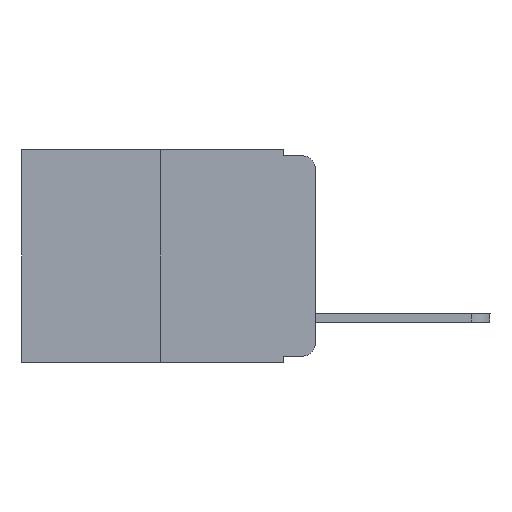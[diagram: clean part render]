
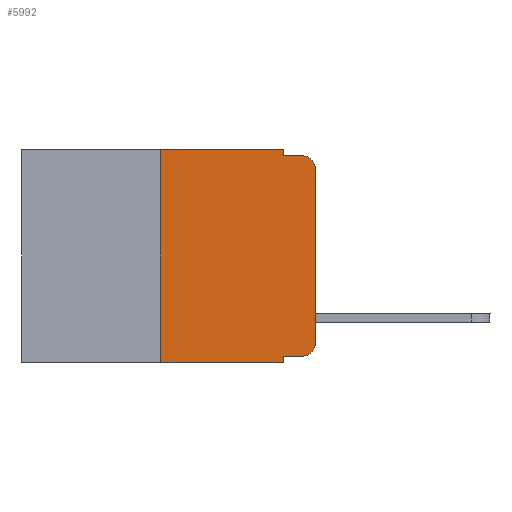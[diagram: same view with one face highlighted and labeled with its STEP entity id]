
A CAD part, left-side view. The second image highlights one B-rep face of the part: STEP entity #5992.
In plain terms, the highlighted planar face has unit normal (-1, 0, 0).
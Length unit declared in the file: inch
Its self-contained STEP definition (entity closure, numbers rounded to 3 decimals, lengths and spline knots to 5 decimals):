
#54 = VECTOR ( 'NONE', #4300, 39.37008 ) ;
#145 = VECTOR ( 'NONE', #15289, 39.37008 ) ;
#254 = PLANE ( 'NONE',  #7755 ) ;
#296 = LINE ( 'NONE', #3203, #15888 ) ;
#339 = VECTOR ( 'NONE', #8221, 39.37008 ) ;
#376 = LINE ( 'NONE', #16861, #54 ) ;
#818 = CARTESIAN_POINT ( 'NONE',  ( 0., 0.051, 0. ) ) ;
#843 = CARTESIAN_POINT ( 'NONE',  ( 0., 0.25, 0. ) ) ;
#1325 = CARTESIAN_POINT ( 'NONE',  ( 0., 0.473, 0. ) ) ;
#1671 = VERTEX_POINT ( 'NONE', #8772 ) ;
#1815 = CARTESIAN_POINT ( 'NONE',  ( 0., 0., 0. ) ) ;
#2217 = VERTEX_POINT ( 'NONE', #7642 ) ;
#2383 = ORIENTED_EDGE ( 'NONE', *, *, #7531, .F. ) ;
#2598 = CARTESIAN_POINT ( 'NONE',  ( 0., 0.02, -0.03 ) ) ;
#2731 = EDGE_CURVE ( 'NONE', #16089, #1671, #296, .T. ) ;
#2764 = CARTESIAN_POINT ( 'NONE',  ( 0., 0.051, -0.333 ) ) ;
#2862 = ORIENTED_EDGE ( 'NONE', *, *, #13841, .F. ) ;
#2972 = ORIENTED_EDGE ( 'NONE', *, *, #16739, .T. ) ;
#2994 = CARTESIAN_POINT ( 'NONE',  ( 0., 0.051, -0.01 ) ) ;
#3203 = CARTESIAN_POINT ( 'NONE',  ( 0., 0.051, -0.333 ) ) ;
#3893 = EDGE_CURVE ( 'NONE', #2217, #14074, #13773, .T. ) ;
#4105 = VERTEX_POINT ( 'NONE', #6702 ) ;
#4200 = CARTESIAN_POINT ( 'NONE',  ( 0., 0., -0.03 ) ) ;
#4300 = DIRECTION ( 'NONE',  ( 0., 0., -1. ) ) ;
#4451 = CARTESIAN_POINT ( 'NONE',  ( 0., 0.473, 0. ) ) ;
#4842 = LINE ( 'NONE', #1815, #11872 ) ;
#4880 = VERTEX_POINT ( 'NONE', #8976 ) ;
#5823 = EDGE_CURVE ( 'NONE', #4105, #11943, #7794, .T. ) ;
#5889 = DIRECTION ( 'NONE',  ( 0., -1., 0. ) ) ;
#5992 = ADVANCED_FACE ( 'NONE', ( #12905 ), #254, .F. ) ;
#6702 = CARTESIAN_POINT ( 'NONE',  ( 0., 0.051, 0. ) ) ;
#6737 = ORIENTED_EDGE ( 'NONE', *, *, #5823, .F. ) ;
#6950 = EDGE_LOOP ( 'NONE', ( #2972, #15024, #8803, #6737, #2862, #14785, #15676, #2383, #9348, #11802 ) ) ;
#6998 = DIRECTION ( 'NONE',  ( 0., 0., -1. ) ) ;
#7228 = DIRECTION ( 'NONE',  ( 0., 0., -1. ) ) ;
#7283 = DIRECTION ( 'NONE',  ( 0., -1., 0. ) ) ;
#7531 = EDGE_CURVE ( 'NONE', #16089, #12881, #376, .T. ) ;
#7642 = CARTESIAN_POINT ( 'NONE',  ( 0., 0.25, -0.343 ) ) ;
#7755 = AXIS2_PLACEMENT_3D ( 'NONE', #4451, #10089, #14267 ) ;
#7794 = LINE ( 'NONE', #818, #145 ) ;
#8005 = EDGE_CURVE ( 'NONE', #11943, #13350, #15561, .T. ) ;
#8221 = DIRECTION ( 'NONE',  ( 0., -1., 0. ) ) ;
#8237 = AXIS2_PLACEMENT_3D ( 'NONE', #8995, #8810, #7228 ) ;
#8254 = AXIS2_PLACEMENT_3D ( 'NONE', #2598, #13702, #6998 ) ;
#8705 = DIRECTION ( 'NONE',  ( 0., -1., 0. ) ) ;
#8756 = VECTOR ( 'NONE', #12595, 39.37008 ) ;
#8772 = CARTESIAN_POINT ( 'NONE',  ( 0., 0.02, -0.333 ) ) ;
#8803 = ORIENTED_EDGE ( 'NONE', *, *, #8005, .F. ) ;
#8810 = DIRECTION ( 'NONE',  ( -1., 0., 0. ) ) ;
#8976 = CARTESIAN_POINT ( 'NONE',  ( 0., 0., -0.313 ) ) ;
#8995 = CARTESIAN_POINT ( 'NONE',  ( 0., 0.02, -0.313 ) ) ;
#9348 = ORIENTED_EDGE ( 'NONE', *, *, #2731, .T. ) ;
#9381 = CARTESIAN_POINT ( 'NONE',  ( 0., 0.051, -0.343 ) ) ;
#9615 = EDGE_CURVE ( 'NONE', #2217, #12881, #16649, .T. ) ;
#9812 = CARTESIAN_POINT ( 'NONE',  ( 0., 0.02, -0.01 ) ) ;
#10089 = DIRECTION ( 'NONE',  ( 1., 0., 0. ) ) ;
#10105 = CARTESIAN_POINT ( 'NONE',  ( 0., 0.051, -0.01 ) ) ;
#10522 = VECTOR ( 'NONE', #7283, 39.37008 ) ;
#11496 = LINE ( 'NONE', #1325, #339 ) ;
#11797 = VERTEX_POINT ( 'NONE', #4200 ) ;
#11802 = ORIENTED_EDGE ( 'NONE', *, *, #13179, .T. ) ;
#11872 = VECTOR ( 'NONE', #14561, 39.37008 ) ;
#11943 = VERTEX_POINT ( 'NONE', #10105 ) ;
#12052 = CIRCLE ( 'NONE', #8237, 0.02 ) ;
#12419 = CARTESIAN_POINT ( 'NONE',  ( 0., 0.25, 0. ) ) ;
#12595 = DIRECTION ( 'NONE',  ( 0., 0., 1. ) ) ;
#12881 = VERTEX_POINT ( 'NONE', #9381 ) ;
#12905 = FACE_OUTER_BOUND ( 'NONE', #6950, .T. ) ;
#13179 = EDGE_CURVE ( 'NONE', #1671, #4880, #12052, .T. ) ;
#13350 = VERTEX_POINT ( 'NONE', #9812 ) ;
#13702 = DIRECTION ( 'NONE',  ( -1., 0., 0. ) ) ;
#13773 = LINE ( 'NONE', #12419, #8756 ) ;
#13833 = EDGE_CURVE ( 'NONE', #11797, #13350, #16144, .T. ) ;
#13841 = EDGE_CURVE ( 'NONE', #14074, #4105, #11496, .T. ) ;
#13964 = VECTOR ( 'NONE', #8705, 39.37008 ) ;
#14074 = VERTEX_POINT ( 'NONE', #843 ) ;
#14267 = DIRECTION ( 'NONE',  ( 0., 0., -1. ) ) ;
#14561 = DIRECTION ( 'NONE',  ( 0., 0., 1. ) ) ;
#14785 = ORIENTED_EDGE ( 'NONE', *, *, #3893, .F. ) ;
#15024 = ORIENTED_EDGE ( 'NONE', *, *, #13833, .T. ) ;
#15289 = DIRECTION ( 'NONE',  ( 0., 0., -1. ) ) ;
#15449 = CARTESIAN_POINT ( 'NONE',  ( 0., 0.473, -0.343 ) ) ;
#15561 = LINE ( 'NONE', #2994, #13964 ) ;
#15676 = ORIENTED_EDGE ( 'NONE', *, *, #9615, .T. ) ;
#15888 = VECTOR ( 'NONE', #5889, 39.37008 ) ;
#16089 = VERTEX_POINT ( 'NONE', #2764 ) ;
#16144 = CIRCLE ( 'NONE', #8254, 0.02 ) ;
#16649 = LINE ( 'NONE', #15449, #10522 ) ;
#16739 = EDGE_CURVE ( 'NONE', #4880, #11797, #4842, .T. ) ;
#16861 = CARTESIAN_POINT ( 'NONE',  ( 0., 0.051, 0. ) ) ;
